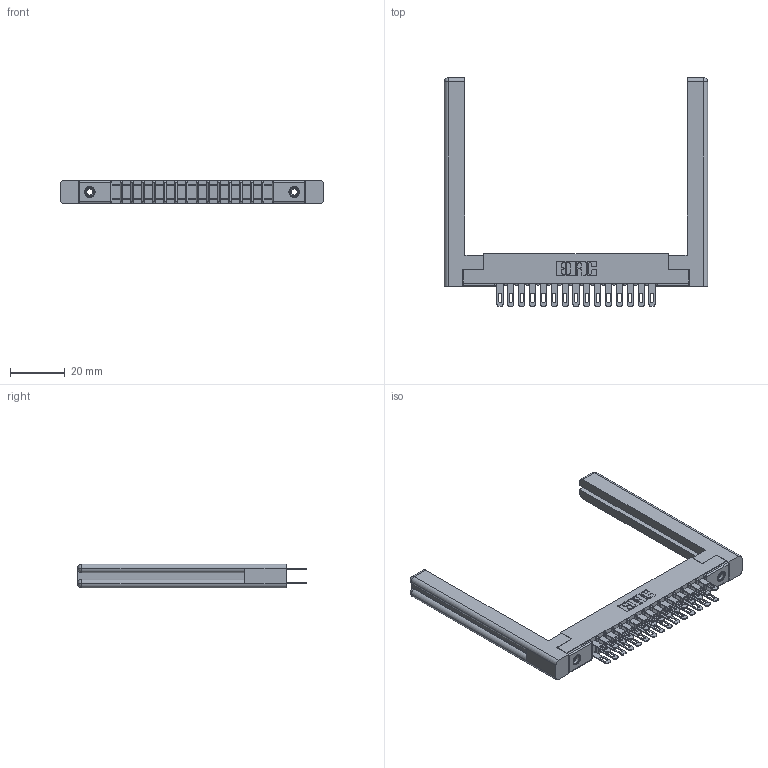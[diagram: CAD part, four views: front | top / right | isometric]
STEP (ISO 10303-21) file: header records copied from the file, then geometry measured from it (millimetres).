
FILE_DESCRIPTION (( 'STEP AP203' ), '1' );
FILE_NAME ('307-030-500-258.STEP', '2019-09-06T00:22:26', ( '' ), ( '' ), 'SwSTEP 2.0', 'SolidWorks 2016', '' );
FILE_SCHEMA (( 'CONFIG_CONTROL_DESIGN' ));
Length unit declared in the file: inch
Products named in the file (5): 307-220-058; 307-030-500-258; 307-290-001_500; 307 Part_.156 Dia Mounting Holes; 345-250-001_345-250-001-102
Assembly tree (35 placements, depth 2):
  307-030-500-258
    307 Part_.156 Dia Mounting Holes
    307-290-001_500  x30
    307-220-058  x2
    345-250-001_345-250-001-102  x2
Bounding box: 96.06 x 83.49 x 8.71 mm (x, y, z)
Volume: 14056.9 mm3; surface area: 16452.8 mm2
Topology: 35 solids, 35 shells, 1656 faces, 4577 edges, 2954 vertices
Faces by surface type: plane 1054, cylinder 546, sphere 32, torus 12, cone 12
Entity records: 19275 total; most frequent: CARTESIAN_POINT 3178, ORIENTED_EDGE 3088, DIRECTION 3084, EDGE_CURVE 1544, LINE 1168, VECTOR 1168, VERTEX_POINT 998, AXIS2_PLACEMENT_3D 958
